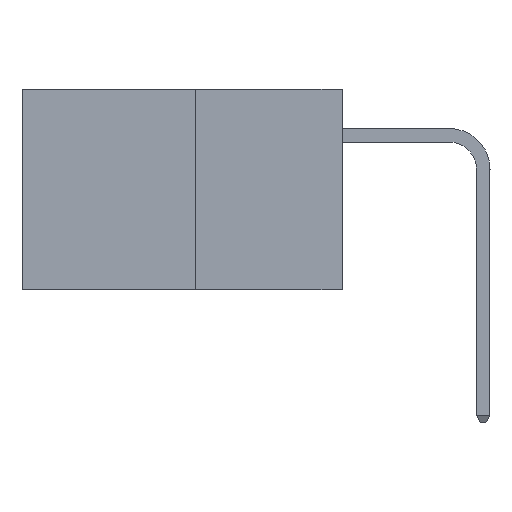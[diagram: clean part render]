
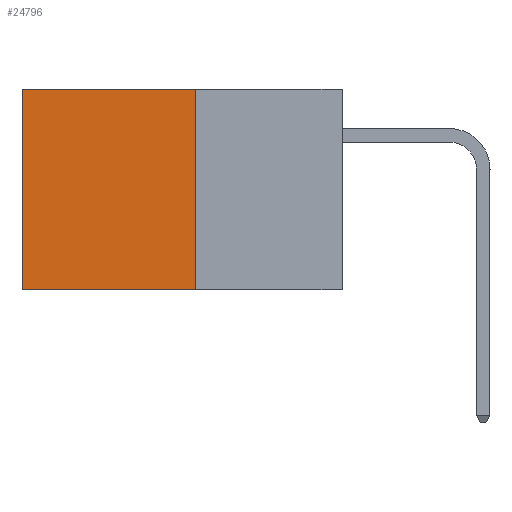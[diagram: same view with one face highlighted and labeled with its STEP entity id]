
A CAD part, left-side view. The second image highlights one B-rep face of the part: STEP entity #24796.
In plain terms, the highlighted planar face has unit normal (-1, 0, 0).
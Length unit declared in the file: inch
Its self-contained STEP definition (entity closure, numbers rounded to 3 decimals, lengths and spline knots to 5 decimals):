
#971 = CARTESIAN_POINT ( 'NONE',  ( 0.277, 0.27, -0.37 ) ) ;
#1336 = LINE ( 'NONE', #21537, #31297 ) ;
#1693 = ORIENTED_EDGE ( 'NONE', *, *, #30784, .F. ) ;
#2149 = DIRECTION ( 'NONE',  ( 0., 1., 0. ) ) ;
#2245 = DIRECTION ( 'NONE',  ( 0., 0., -1. ) ) ;
#2256 = CARTESIAN_POINT ( 'NONE',  ( 0.277, 0.27, -0.37 ) ) ;
#2654 = ORIENTED_EDGE ( 'NONE', *, *, #13752, .F. ) ;
#2709 = VECTOR ( 'NONE', #10597, 39.37008 ) ;
#5803 = VECTOR ( 'NONE', #26538, 39.37008 ) ;
#8907 = VERTEX_POINT ( 'NONE', #15473 ) ;
#9853 = LINE ( 'NONE', #971, #2709 ) ;
#9937 = VERTEX_POINT ( 'NONE', #20361 ) ;
#10597 = DIRECTION ( 'NONE',  ( 0., 0., -1. ) ) ;
#10841 = VECTOR ( 'NONE', #2245, 39.37008 ) ;
#11361 = FACE_OUTER_BOUND ( 'NONE', #21416, .T. ) ;
#11648 = DIRECTION ( 'NONE',  ( 0., 0., -1. ) ) ;
#13752 = EDGE_CURVE ( 'NONE', #29408, #14626, #9853, .T. ) ;
#14304 = CARTESIAN_POINT ( 'NONE',  ( 0.277, 0.59, -0.37 ) ) ;
#14626 = VERTEX_POINT ( 'NONE', #19042 ) ;
#15473 = CARTESIAN_POINT ( 'NONE',  ( 0.277, 0.59, 0. ) ) ;
#16306 = CARTESIAN_POINT ( 'NONE',  ( 0.277, 0.27, 0. ) ) ;
#16446 = PLANE ( 'NONE',  #30985 ) ;
#19042 = CARTESIAN_POINT ( 'NONE',  ( 0.277, 0.27, -0.37 ) ) ;
#19355 = EDGE_CURVE ( 'NONE', #29408, #8907, #1336, .T. ) ;
#20227 = LINE ( 'NONE', #2256, #5803 ) ;
#20361 = CARTESIAN_POINT ( 'NONE',  ( 0.277, 0.59, -0.37 ) ) ;
#21341 = EDGE_CURVE ( 'NONE', #8907, #9937, #30991, .T. ) ;
#21416 = EDGE_LOOP ( 'NONE', ( #29266, #1693, #2654, #30977 ) ) ;
#21537 = CARTESIAN_POINT ( 'NONE',  ( 0.277, 0.27, 0. ) ) ;
#24796 = ADVANCED_FACE ( 'NONE', ( #11361 ), #16446, .F. ) ;
#26214 = DIRECTION ( 'NONE',  ( 1., 0., 0. ) ) ;
#26538 = DIRECTION ( 'NONE',  ( 0., 1., 0. ) ) ;
#29266 = ORIENTED_EDGE ( 'NONE', *, *, #21341, .T. ) ;
#29408 = VERTEX_POINT ( 'NONE', #16306 ) ;
#30784 = EDGE_CURVE ( 'NONE', #14626, #9937, #20227, .T. ) ;
#30977 = ORIENTED_EDGE ( 'NONE', *, *, #19355, .T. ) ;
#30985 = AXIS2_PLACEMENT_3D ( 'NONE', #30999, #26214, #11648 ) ;
#30991 = LINE ( 'NONE', #14304, #10841 ) ;
#30999 = CARTESIAN_POINT ( 'NONE',  ( 0.277, 0.27, -0.37 ) ) ;
#31297 = VECTOR ( 'NONE', #2149, 39.37008 ) ;
